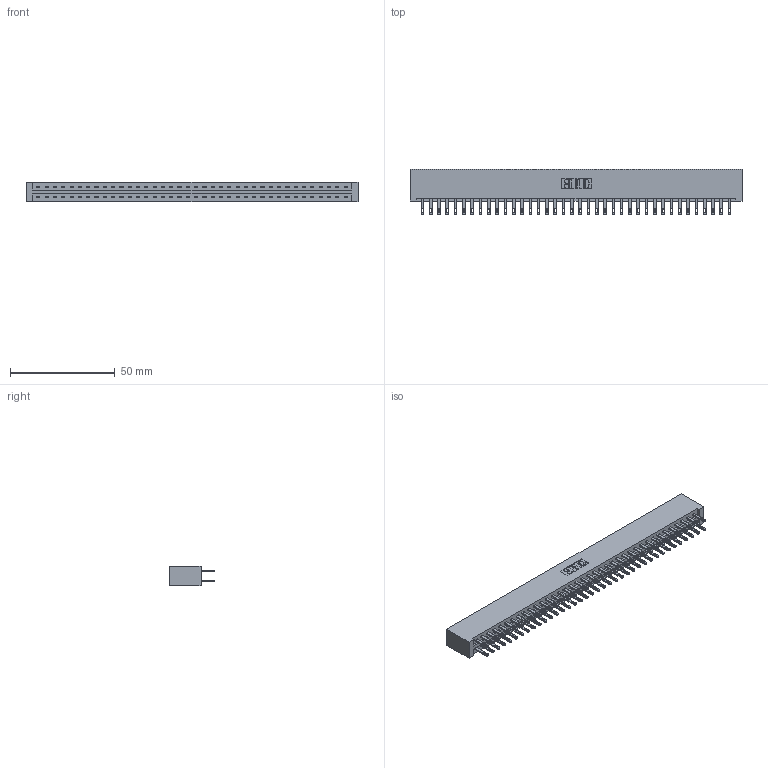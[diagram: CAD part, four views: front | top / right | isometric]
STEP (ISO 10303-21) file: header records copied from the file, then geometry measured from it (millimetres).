
FILE_DESCRIPTION (( 'STEP AP203' ), '1' );
FILE_NAME ('887-076-500-201.STEP', '2020-09-21T03:48:34', ( '' ), ( '' ), 'SwSTEP 2.0', 'SolidWorks 2020', '' );
FILE_SCHEMA (( 'CONFIG_CONTROL_DESIGN' ));
Length unit declared in the file: inch
Products named in the file (3): 345-292-001_345-293-100; 837 Part_No Mounting Lugs; 887-076-500-201
Assembly tree (77 placements, depth 2):
  887-076-500-201
    837 Part_No Mounting Lugs
    345-292-001_345-293-100  x76
Bounding box: 158.45 x 21.85 x 9.4 mm (x, y, z)
Volume: 17637.9 mm3; surface area: 20800.3 mm2
Topology: 77 solids, 77 shells, 3906 faces, 11915 edges, 7942 vertices
Faces by surface type: plane 2498, cylinder 1408
Entity records: 29633 total; most frequent: CARTESIAN_POINT 4994, ORIENTED_EDGE 4930, DIRECTION 4249, EDGE_CURVE 2465, LINE 2341, VECTOR 2341, VERTEX_POINT 1642, AXIS2_PLACEMENT_3D 954
